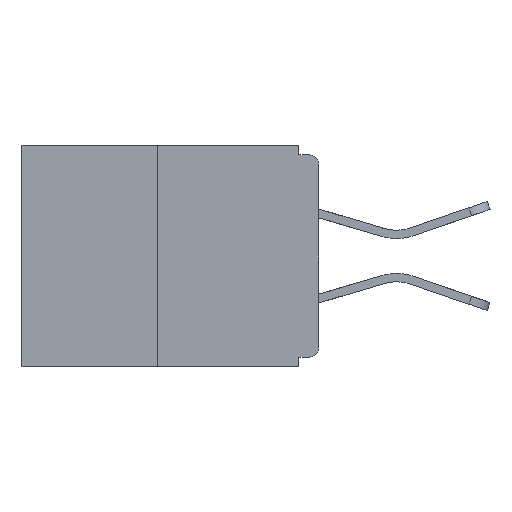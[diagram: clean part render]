
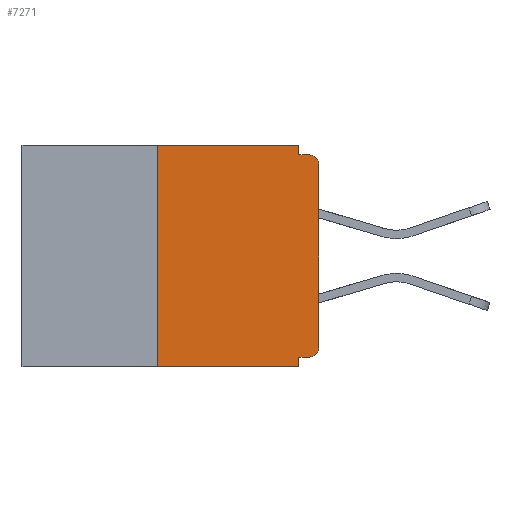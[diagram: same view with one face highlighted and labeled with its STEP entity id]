
A CAD part, left-side view. The second image highlights one B-rep face of the part: STEP entity #7271.
In plain terms, the highlighted planar face has unit normal (-1, 0, 0).
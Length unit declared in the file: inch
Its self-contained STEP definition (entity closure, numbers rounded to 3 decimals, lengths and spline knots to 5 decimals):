
#935 = EDGE_CURVE ( 'NONE', #7169, #1742, #15705, .T. ) ;
#1192 = LINE ( 'NONE', #10971, #15971 ) ;
#1742 = VERTEX_POINT ( 'NONE', #8172 ) ;
#1852 = DIRECTION ( 'NONE',  ( -1., 0., 0. ) ) ;
#1884 = VERTEX_POINT ( 'NONE', #20355 ) ;
#2036 = VECTOR ( 'NONE', #11249, 39.37008 ) ;
#2095 = EDGE_LOOP ( 'NONE', ( #12795, #7060, #15959, #2647, #2415, #5054, #13236, #18556, #12949, #17669 ) ) ;
#2166 = CARTESIAN_POINT ( 'NONE',  ( 0., 0.015, -0.015 ) ) ;
#2333 = CARTESIAN_POINT ( 'NONE',  ( 0., 0., -0.313 ) ) ;
#2339 = CARTESIAN_POINT ( 'NONE',  ( 0., 0.031, -0.343 ) ) ;
#2415 = ORIENTED_EDGE ( 'NONE', *, *, #8398, .F. ) ;
#2574 = DIRECTION ( 'NONE',  ( 0., 0., -1. ) ) ;
#2647 = ORIENTED_EDGE ( 'NONE', *, *, #12016, .F. ) ;
#2700 = DIRECTION ( 'NONE',  ( 0., -1., 0. ) ) ;
#2870 = VECTOR ( 'NONE', #10975, 39.37008 ) ;
#3204 = CARTESIAN_POINT ( 'NONE',  ( 0., 0.031, 0. ) ) ;
#3502 = DIRECTION ( 'NONE',  ( 0., 0., -1. ) ) ;
#3580 = CARTESIAN_POINT ( 'NONE',  ( 0., 0.015, -0.03 ) ) ;
#4019 = CARTESIAN_POINT ( 'NONE',  ( 0., 0.031, -0.343 ) ) ;
#4370 = LINE ( 'NONE', #3204, #2036 ) ;
#4391 = CARTESIAN_POINT ( 'NONE',  ( 0., 0.015, -0.313 ) ) ;
#4669 = FACE_OUTER_BOUND ( 'NONE', #2095, .T. ) ;
#4820 = VERTEX_POINT ( 'NONE', #9640 ) ;
#5054 = ORIENTED_EDGE ( 'NONE', *, *, #20700, .T. ) ;
#5069 = VECTOR ( 'NONE', #12391, 39.37008 ) ;
#5084 = AXIS2_PLACEMENT_3D ( 'NONE', #4391, #18876, #10784 ) ;
#5096 = CARTESIAN_POINT ( 'NONE',  ( 0., 0., 0. ) ) ;
#5295 = CARTESIAN_POINT ( 'NONE',  ( 0., 0.25, 0. ) ) ;
#5549 = AXIS2_PLACEMENT_3D ( 'NONE', #3580, #1852, #3502 ) ;
#5592 = CARTESIAN_POINT ( 'NONE',  ( 0., 0., -0.015 ) ) ;
#5814 = CARTESIAN_POINT ( 'NONE',  ( 0., 0.46, 0. ) ) ;
#6432 = VERTEX_POINT ( 'NONE', #4019 ) ;
#7060 = ORIENTED_EDGE ( 'NONE', *, *, #20294, .F. ) ;
#7087 = VECTOR ( 'NONE', #18087, 39.37008 ) ;
#7156 = CIRCLE ( 'NONE', #5549, 0.015 ) ;
#7169 = VERTEX_POINT ( 'NONE', #2333 ) ;
#7235 = LINE ( 'NONE', #20622, #2870 ) ;
#7271 = ADVANCED_FACE ( 'NONE', ( #4669 ), #13913, .F. ) ;
#8172 = CARTESIAN_POINT ( 'NONE',  ( 0., 0., -0.03 ) ) ;
#8398 = EDGE_CURVE ( 'NONE', #4820, #8518, #16054, .T. ) ;
#8518 = VERTEX_POINT ( 'NONE', #16415 ) ;
#9207 = CARTESIAN_POINT ( 'NONE',  ( 0., 0.25, -0.343 ) ) ;
#9290 = VECTOR ( 'NONE', #10488, 39.37008 ) ;
#9640 = CARTESIAN_POINT ( 'NONE',  ( 0., 0.015, -0.328 ) ) ;
#10087 = LINE ( 'NONE', #2339, #9290 ) ;
#10454 = EDGE_CURVE ( 'NONE', #16424, #6432, #1192, .T. ) ;
#10488 = DIRECTION ( 'NONE',  ( 0., 0., -1. ) ) ;
#10554 = VERTEX_POINT ( 'NONE', #18291 ) ;
#10784 = DIRECTION ( 'NONE',  ( 0., 0., -1. ) ) ;
#10971 = CARTESIAN_POINT ( 'NONE',  ( 0., 0.46, -0.343 ) ) ;
#10975 = DIRECTION ( 'NONE',  ( 0., -1., 0. ) ) ;
#11214 = VECTOR ( 'NONE', #19264, 39.37008 ) ;
#11239 = CIRCLE ( 'NONE', #5084, 0.015 ) ;
#11249 = DIRECTION ( 'NONE',  ( 0., 0., -1. ) ) ;
#12016 = EDGE_CURVE ( 'NONE', #8518, #6432, #10087, .T. ) ;
#12391 = DIRECTION ( 'NONE',  ( 0., -1., 0. ) ) ;
#12795 = ORIENTED_EDGE ( 'NONE', *, *, #19929, .F. ) ;
#12949 = ORIENTED_EDGE ( 'NONE', *, *, #17336, .F. ) ;
#13236 = ORIENTED_EDGE ( 'NONE', *, *, #935, .T. ) ;
#13312 = VERTEX_POINT ( 'NONE', #2166 ) ;
#13808 = LINE ( 'NONE', #18396, #19924 ) ;
#13913 = PLANE ( 'NONE',  #15648 ) ;
#14106 = EDGE_CURVE ( 'NONE', #1884, #10554, #4370, .T. ) ;
#15500 = EDGE_CURVE ( 'NONE', #1742, #13312, #7156, .T. ) ;
#15648 = AXIS2_PLACEMENT_3D ( 'NONE', #5814, #17181, #2574 ) ;
#15705 = LINE ( 'NONE', #5096, #7087 ) ;
#15959 = ORIENTED_EDGE ( 'NONE', *, *, #10454, .T. ) ;
#15971 = VECTOR ( 'NONE', #2700, 39.37008 ) ;
#15990 = CARTESIAN_POINT ( 'NONE',  ( 0., 0., -0.328 ) ) ;
#16054 = LINE ( 'NONE', #15990, #11214 ) ;
#16415 = CARTESIAN_POINT ( 'NONE',  ( 0., 0.031, -0.328 ) ) ;
#16424 = VERTEX_POINT ( 'NONE', #9207 ) ;
#16838 = DIRECTION ( 'NONE',  ( 0., 0., 1. ) ) ;
#17181 = DIRECTION ( 'NONE',  ( 1., 0., 0. ) ) ;
#17336 = EDGE_CURVE ( 'NONE', #10554, #13312, #18024, .T. ) ;
#17466 = VERTEX_POINT ( 'NONE', #5295 ) ;
#17669 = ORIENTED_EDGE ( 'NONE', *, *, #14106, .F. ) ;
#18024 = LINE ( 'NONE', #5592, #5069 ) ;
#18087 = DIRECTION ( 'NONE',  ( 0., 0., 1. ) ) ;
#18291 = CARTESIAN_POINT ( 'NONE',  ( 0., 0.031, -0.015 ) ) ;
#18396 = CARTESIAN_POINT ( 'NONE',  ( 0., 0.25, 0. ) ) ;
#18556 = ORIENTED_EDGE ( 'NONE', *, *, #15500, .T. ) ;
#18876 = DIRECTION ( 'NONE',  ( -1., 0., 0. ) ) ;
#19264 = DIRECTION ( 'NONE',  ( 0., 1., 0. ) ) ;
#19924 = VECTOR ( 'NONE', #16838, 39.37008 ) ;
#19929 = EDGE_CURVE ( 'NONE', #17466, #1884, #7235, .T. ) ;
#20294 = EDGE_CURVE ( 'NONE', #16424, #17466, #13808, .T. ) ;
#20355 = CARTESIAN_POINT ( 'NONE',  ( 0., 0.031, 0. ) ) ;
#20622 = CARTESIAN_POINT ( 'NONE',  ( 0., 0.46, 0. ) ) ;
#20700 = EDGE_CURVE ( 'NONE', #4820, #7169, #11239, .T. ) ;
